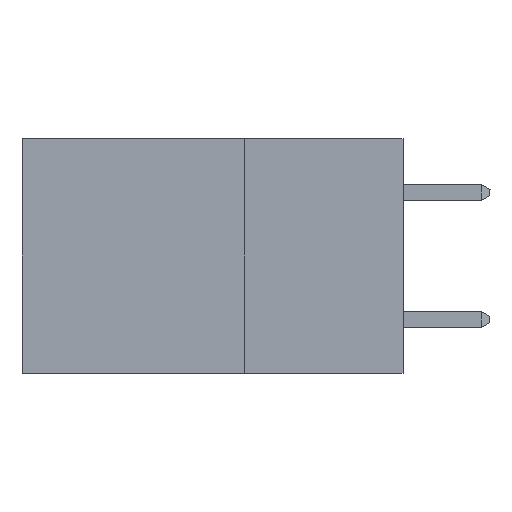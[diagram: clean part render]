
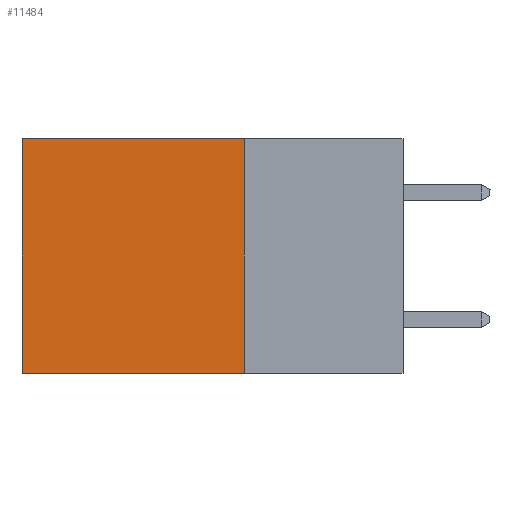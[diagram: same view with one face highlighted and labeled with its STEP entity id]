
A CAD part, left-side view. The second image highlights one B-rep face of the part: STEP entity #11484.
In plain terms, the highlighted planar face has unit normal (-1, 0, 0).
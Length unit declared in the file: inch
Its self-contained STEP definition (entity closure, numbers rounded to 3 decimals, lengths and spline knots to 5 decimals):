
#148 = CARTESIAN_POINT ( 'NONE',  ( 0.2875, 0.25, 0. ) ) ;
#244 = VERTEX_POINT ( 'NONE', #17897 ) ;
#304 = VECTOR ( 'NONE', #16835, 39.37008 ) ;
#1368 = ORIENTED_EDGE ( 'NONE', *, *, #10872, .T. ) ;
#1494 = EDGE_LOOP ( 'NONE', ( #15672, #4968, #2927, #1368 ) ) ;
#1503 = CARTESIAN_POINT ( 'NONE',  ( 0.2875, 0.25, 0. ) ) ;
#2414 = CARTESIAN_POINT ( 'NONE',  ( 0.2875, 0.6, 0. ) ) ;
#2927 = ORIENTED_EDGE ( 'NONE', *, *, #11581, .F. ) ;
#3212 = LINE ( 'NONE', #15550, #17353 ) ;
#3532 = AXIS2_PLACEMENT_3D ( 'NONE', #11681, #16012, #15329 ) ;
#3708 = DIRECTION ( 'NONE',  ( 0., 1., 0. ) ) ;
#4060 = FACE_OUTER_BOUND ( 'NONE', #1494, .T. ) ;
#4911 = CARTESIAN_POINT ( 'NONE',  ( 0.2875, 0.25, -0.37 ) ) ;
#4968 = ORIENTED_EDGE ( 'NONE', *, *, #6260, .F. ) ;
#5564 = CARTESIAN_POINT ( 'NONE',  ( 0.2875, 0.6, 0. ) ) ;
#6253 = LINE ( 'NONE', #4911, #16225 ) ;
#6260 = EDGE_CURVE ( 'NONE', #244, #12536, #6253, .T. ) ;
#7207 = LINE ( 'NONE', #5564, #14576 ) ;
#10112 = DIRECTION ( 'NONE',  ( 0., 1., 0. ) ) ;
#10153 = EDGE_CURVE ( 'NONE', #10442, #12536, #7207, .T. ) ;
#10259 = PLANE ( 'NONE',  #3532 ) ;
#10442 = VERTEX_POINT ( 'NONE', #2414 ) ;
#10872 = EDGE_CURVE ( 'NONE', #18042, #10442, #3212, .T. ) ;
#11430 = CARTESIAN_POINT ( 'NONE',  ( 0.2875, 0.6, -0.37 ) ) ;
#11484 = ADVANCED_FACE ( 'NONE', ( #4060 ), #10259, .F. ) ;
#11485 = LINE ( 'NONE', #1503, #304 ) ;
#11581 = EDGE_CURVE ( 'NONE', #18042, #244, #11485, .T. ) ;
#11681 = CARTESIAN_POINT ( 'NONE',  ( 0.2875, 0.25, 0. ) ) ;
#12536 = VERTEX_POINT ( 'NONE', #11430 ) ;
#14576 = VECTOR ( 'NONE', #18033, 39.37008 ) ;
#15329 = DIRECTION ( 'NONE',  ( 0., 0., -1. ) ) ;
#15550 = CARTESIAN_POINT ( 'NONE',  ( 0.2875, 0.25, 0. ) ) ;
#15672 = ORIENTED_EDGE ( 'NONE', *, *, #10153, .T. ) ;
#16012 = DIRECTION ( 'NONE',  ( 1., 0., 0. ) ) ;
#16225 = VECTOR ( 'NONE', #3708, 39.37008 ) ;
#16835 = DIRECTION ( 'NONE',  ( 0., 0., -1. ) ) ;
#17353 = VECTOR ( 'NONE', #10112, 39.37008 ) ;
#17897 = CARTESIAN_POINT ( 'NONE',  ( 0.2875, 0.25, -0.37 ) ) ;
#18033 = DIRECTION ( 'NONE',  ( 0., 0., -1. ) ) ;
#18042 = VERTEX_POINT ( 'NONE', #148 ) ;
